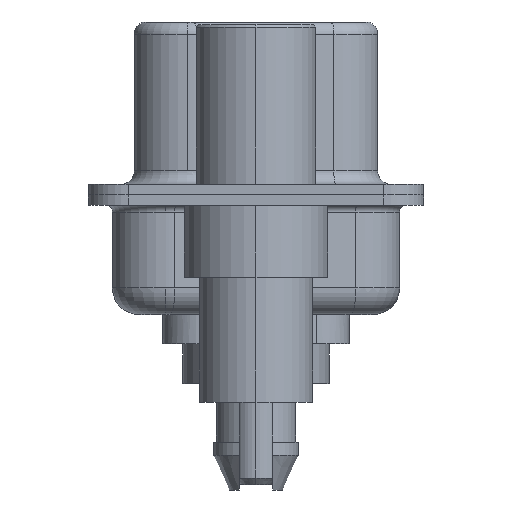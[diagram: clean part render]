
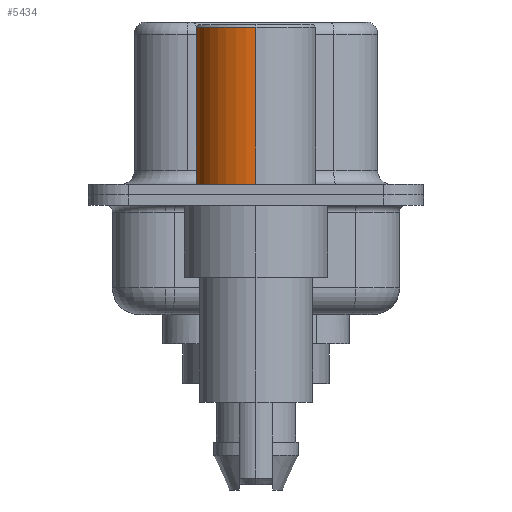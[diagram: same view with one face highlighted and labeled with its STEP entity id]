
A CAD part, left-side view. The second image highlights one B-rep face of the part: STEP entity #5434.
In plain terms, the highlighted cylindrical face has radius 2.25 mm (diameter 4.5 mm), a partial arc.
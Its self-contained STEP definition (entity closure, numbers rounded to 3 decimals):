
#63 = VERTEX_POINT ( 'NONE', #3295 ) ;
#66 = CARTESIAN_POINT ( 'NONE',  ( -2.25, 0., 6.3 ) ) ;
#529 = VERTEX_POINT ( 'NONE', #9059 ) ;
#742 = AXIS2_PLACEMENT_3D ( 'NONE', #3860, #13531, #5261 ) ;
#1120 = VECTOR ( 'NONE', #4952, 1000. ) ;
#2232 = FACE_OUTER_BOUND ( 'NONE', #12685, .T. ) ;
#2245 = DIRECTION ( 'NONE',  ( 0., 0., 1. ) ) ;
#2284 = EDGE_CURVE ( 'NONE', #529, #12357, #9941, .T. ) ;
#3295 = CARTESIAN_POINT ( 'NONE',  ( 2.25, 0., 6.3 ) ) ;
#3486 = CARTESIAN_POINT ( 'NONE',  ( 2.25, 0., 0.581 ) ) ;
#3860 = CARTESIAN_POINT ( 'NONE',  ( 0., 0., 0.4 ) ) ;
#4056 = DIRECTION ( 'NONE',  ( 0., 0., 1. ) ) ;
#4952 = DIRECTION ( 'NONE',  ( 0., 0., 1. ) ) ;
#5098 = ORIENTED_EDGE ( 'NONE', *, *, #13488, .F. ) ;
#5261 = DIRECTION ( 'NONE',  ( 1., 0., 0. ) ) ;
#5434 = ADVANCED_FACE ( 'NONE', ( #2232 ), #9164, .T. ) ;
#6318 = VECTOR ( 'NONE', #2245, 1000. ) ;
#7699 = CARTESIAN_POINT ( 'NONE',  ( 0., 0., 6.3 ) ) ;
#8321 = VERTEX_POINT ( 'NONE', #14601 ) ;
#9059 = CARTESIAN_POINT ( 'NONE',  ( -2.25, 0., 0.4 ) ) ;
#9083 = DIRECTION ( 'NONE',  ( 1., 0., 0. ) ) ;
#9164 = CYLINDRICAL_SURFACE ( 'NONE', #9712, 2.25 ) ;
#9712 = AXIS2_PLACEMENT_3D ( 'NONE', #12339, #4056, #10931 ) ;
#9787 = EDGE_CURVE ( 'NONE', #8321, #529, #16748, .T. ) ;
#9941 = LINE ( 'NONE', #16235, #6318 ) ;
#10909 = ORIENTED_EDGE ( 'NONE', *, *, #9787, .T. ) ;
#10931 = DIRECTION ( 'NONE',  ( 1., 0., 0. ) ) ;
#11111 = AXIS2_PLACEMENT_3D ( 'NONE', #7699, #17324, #9083 ) ;
#11219 = EDGE_CURVE ( 'NONE', #8321, #63, #15383, .T. ) ;
#12339 = CARTESIAN_POINT ( 'NONE',  ( 0., 0., 0.581 ) ) ;
#12357 = VERTEX_POINT ( 'NONE', #66 ) ;
#12685 = EDGE_LOOP ( 'NONE', ( #10909, #14888, #5098, #16057 ) ) ;
#13488 = EDGE_CURVE ( 'NONE', #63, #12357, #14465, .T. ) ;
#13531 = DIRECTION ( 'NONE',  ( 0., 0., 1. ) ) ;
#14465 = CIRCLE ( 'NONE', #11111, 2.25 ) ;
#14601 = CARTESIAN_POINT ( 'NONE',  ( 2.25, 0., 0.4 ) ) ;
#14888 = ORIENTED_EDGE ( 'NONE', *, *, #2284, .T. ) ;
#15383 = LINE ( 'NONE', #3486, #1120 ) ;
#16057 = ORIENTED_EDGE ( 'NONE', *, *, #11219, .F. ) ;
#16235 = CARTESIAN_POINT ( 'NONE',  ( -2.25, 0., 0.581 ) ) ;
#16748 = CIRCLE ( 'NONE', #742, 2.25 ) ;
#17324 = DIRECTION ( 'NONE',  ( 0., 0., 1. ) ) ;
